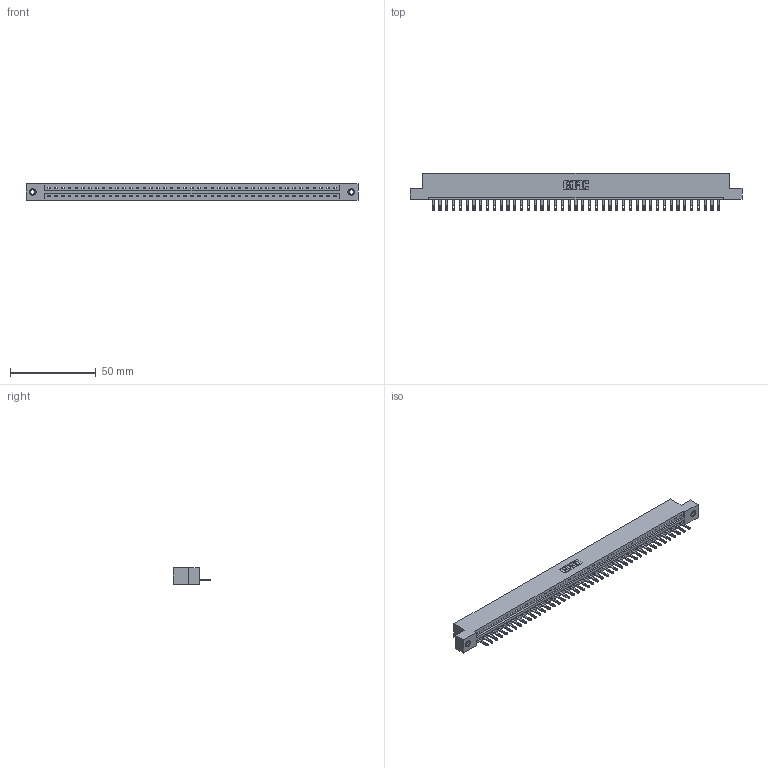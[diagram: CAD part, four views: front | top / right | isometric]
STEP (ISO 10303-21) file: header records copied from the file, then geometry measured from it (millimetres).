
FILE_DESCRIPTION (( 'STEP AP203' ), '1' );
FILE_NAME ('887-043-500-107.STEP', '2020-09-21T00:17:10', ( '' ), ( '' ), 'SwSTEP 2.0', 'SolidWorks 2020', '' );
FILE_SCHEMA (( 'CONFIG_CONTROL_DESIGN' ));
Length unit declared in the file: inch
Products named in the file (4): 345-292-001_345-293-100; 837 Part_Flush Mounting Lugs - 0.156 Dia-TI; 345-250-001_345-250-005-103; 887-043-500-107
Assembly tree (46 placements, depth 2):
  887-043-500-107
    837 Part_Flush Mounting Lugs - 0.156 Dia-TI
    345-292-001_345-293-100  x43
    345-250-001_345-250-005-103  x2
Bounding box: 193.4 x 21.85 x 9.4 mm (x, y, z)
Volume: 20125.8 mm3; surface area: 20944.1 mm2
Topology: 46 solids, 46 shells, 2668 faces, 8187 edges, 5450 vertices
Faces by surface type: plane 1822, cylinder 830, cone 12, torus 4
Entity records: 32950 total; most frequent: CARTESIAN_POINT 5718, ORIENTED_EDGE 5690, DIRECTION 4845, EDGE_CURVE 2845, VECTOR 2693, LINE 2693, VERTEX_POINT 1892, AXIS2_PLACEMENT_3D 1076
